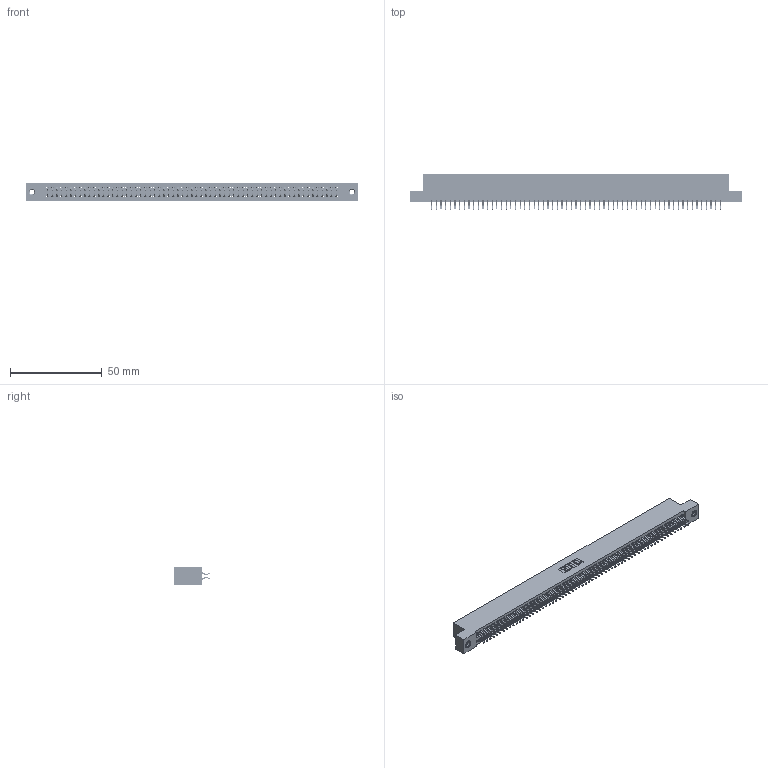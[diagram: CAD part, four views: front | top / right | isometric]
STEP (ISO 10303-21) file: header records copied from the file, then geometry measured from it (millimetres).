
FILE_DESCRIPTION (( 'STEP AP203' ), '1' );
FILE_NAME ('345-126-556-207.STEP', '2018-10-19T17:24:00', ( '' ), ( '' ), 'SwSTEP 2.0', 'SolidWorks 2016', '' );
FILE_SCHEMA (( 'CONFIG_CONTROL_DESIGN' ));
Length unit declared in the file: inch
Products named in the file (4): 345-126-556-207; 345-250-001_345-250-005-103; 345-292-001_556 Tail; 345 Part_Flush Mounting Lugs - 0.156 Dia-TI
Assembly tree (129 placements, depth 2):
  345-126-556-207
    345 Part_Flush Mounting Lugs - 0.156 Dia-TI
    345-292-001_556 Tail  x126
    345-250-001_345-250-005-103  x2
Bounding box: 181.23 x 19.24 x 9.4 mm (x, y, z)
Volume: 17781.2 mm3; surface area: 26607.9 mm2
Topology: 129 solids, 129 shells, 7242 faces, 21519 edges, 14170 vertices
Faces by surface type: plane 4774, cylinder 2452, cone 12, torus 4
Entity records: 48010 total; most frequent: CARTESIAN_POINT 8023, ORIENTED_EDGE 7938, DIRECTION 7063, EDGE_CURVE 3969, LINE 3557, VECTOR 3557, VERTEX_POINT 2640, AXIS2_PLACEMENT_3D 1753
